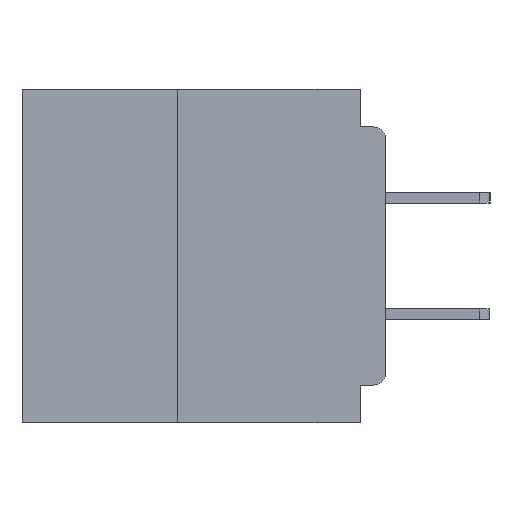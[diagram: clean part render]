
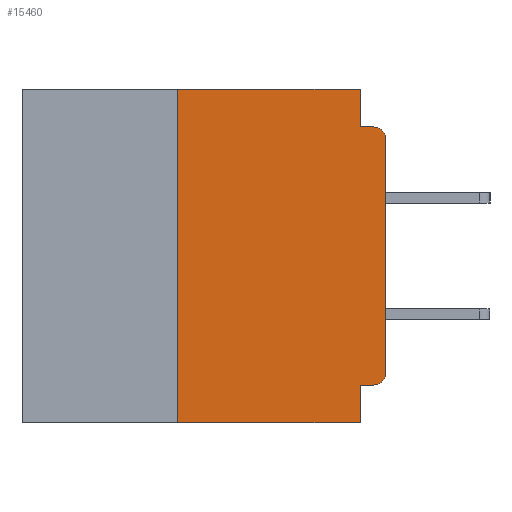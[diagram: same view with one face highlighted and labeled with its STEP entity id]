
A CAD part, left-side view. The second image highlights one B-rep face of the part: STEP entity #15460.
In plain terms, the highlighted planar face has unit normal (-1, 0, 0).
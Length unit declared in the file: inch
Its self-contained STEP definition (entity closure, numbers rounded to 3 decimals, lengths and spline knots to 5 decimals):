
#639 = EDGE_CURVE ( 'NONE', #4602, #40217, #16367, .T. ) ;
#1851 = ORIENTED_EDGE ( 'NONE', *, *, #38420, .F. ) ;
#2623 = LINE ( 'NONE', #29230, #11467 ) ;
#2652 = CARTESIAN_POINT ( 'NONE',  ( 0., 0.031, 0. ) ) ;
#2675 = CARTESIAN_POINT ( 'NONE',  ( 0., 0.015, -0.34 ) ) ;
#3031 = EDGE_CURVE ( 'NONE', #53284, #5341, #20967, .T. ) ;
#3651 = DIRECTION ( 'NONE',  ( 0., -1., 0. ) ) ;
#3928 = PLANE ( 'NONE',  #62300 ) ;
#4035 = DIRECTION ( 'NONE',  ( 0., 0., -1. ) ) ;
#4602 = VERTEX_POINT ( 'NONE', #41053 ) ;
#5341 = VERTEX_POINT ( 'NONE', #62107 ) ;
#5987 = ORIENTED_EDGE ( 'NONE', *, *, #14786, .F. ) ;
#6635 = ORIENTED_EDGE ( 'NONE', *, *, #27034, .F. ) ;
#7859 = DIRECTION ( 'NONE',  ( 0., 0., -1. ) ) ;
#7872 = EDGE_CURVE ( 'NONE', #63508, #13340, #45457, .T. ) ;
#8539 = DIRECTION ( 'NONE',  ( 0., 1., 0. ) ) ;
#9105 = DIRECTION ( 'NONE',  ( 0., 0., -1. ) ) ;
#9615 = LINE ( 'NONE', #51206, #62433 ) ;
#10127 = CARTESIAN_POINT ( 'NONE',  ( 0., 0.031, -0.4 ) ) ;
#11467 = VECTOR ( 'NONE', #3651, 39.37008 ) ;
#11957 = VECTOR ( 'NONE', #20599, 39.37008 ) ;
#12741 = CARTESIAN_POINT ( 'NONE',  ( 0., 0.25, -0.4 ) ) ;
#13340 = VERTEX_POINT ( 'NONE', #47732 ) ;
#14077 = CARTESIAN_POINT ( 'NONE',  ( 0., 0.437, 0. ) ) ;
#14786 = EDGE_CURVE ( 'NONE', #63508, #59188, #64488, .T. ) ;
#15460 = ADVANCED_FACE ( 'NONE', ( #37426 ), #3928, .F. ) ;
#15581 = VECTOR ( 'NONE', #4035, 39.37008 ) ;
#16317 = LINE ( 'NONE', #64250, #55476 ) ;
#16367 = LINE ( 'NONE', #40105, #26764 ) ;
#17853 = ORIENTED_EDGE ( 'NONE', *, *, #26024, .T. ) ;
#18044 = VECTOR ( 'NONE', #45025, 39.37008 ) ;
#18517 = DIRECTION ( 'NONE',  ( 0., 0., -1. ) ) ;
#18874 = VERTEX_POINT ( 'NONE', #64544 ) ;
#18918 = AXIS2_PLACEMENT_3D ( 'NONE', #51100, #20511, #56238 ) ;
#19669 = EDGE_CURVE ( 'NONE', #59188, #24117, #22003, .T. ) ;
#20363 = ORIENTED_EDGE ( 'NONE', *, *, #22897, .T. ) ;
#20511 = DIRECTION ( 'NONE',  ( -1., 0., 0. ) ) ;
#20599 = DIRECTION ( 'NONE',  ( 0., -1., 0. ) ) ;
#20967 = CIRCLE ( 'NONE', #18918, 0.015 ) ;
#22003 = LINE ( 'NONE', #45058, #15581 ) ;
#22897 = EDGE_CURVE ( 'NONE', #30338, #24117, #63167, .T. ) ;
#22945 = CARTESIAN_POINT ( 'NONE',  ( 0., 0.015, -0.355 ) ) ;
#24117 = VERTEX_POINT ( 'NONE', #10127 ) ;
#25753 = DIRECTION ( 'NONE',  ( 0., 0., 1. ) ) ;
#26024 = EDGE_CURVE ( 'NONE', #13340, #53284, #58818, .T. ) ;
#26764 = VECTOR ( 'NONE', #40774, 39.37008 ) ;
#26951 = EDGE_CURVE ( 'NONE', #40217, #18874, #16317, .T. ) ;
#27034 = EDGE_CURVE ( 'NONE', #18874, #5341, #2623, .T. ) ;
#29230 = CARTESIAN_POINT ( 'NONE',  ( 0., 0., -0.045 ) ) ;
#30338 = VERTEX_POINT ( 'NONE', #12741 ) ;
#30377 = CARTESIAN_POINT ( 'NONE',  ( 0., 0., -0.06 ) ) ;
#34748 = ORIENTED_EDGE ( 'NONE', *, *, #639, .F. ) ;
#34998 = AXIS2_PLACEMENT_3D ( 'NONE', #2675, #38575, #7859 ) ;
#37426 = FACE_OUTER_BOUND ( 'NONE', #39822, .T. ) ;
#38420 = EDGE_CURVE ( 'NONE', #30338, #4602, #9615, .T. ) ;
#38575 = DIRECTION ( 'NONE',  ( -1., 0., 0. ) ) ;
#39017 = VECTOR ( 'NONE', #8539, 39.37008 ) ;
#39250 = CARTESIAN_POINT ( 'NONE',  ( 0., 0., -0.355 ) ) ;
#39822 = EDGE_LOOP ( 'NONE', ( #17853, #42738, #6635, #40343, #34748, #1851, #20363, #43602, #5987, #46840 ) ) ;
#39840 = DIRECTION ( 'NONE',  ( 1., 0., 0. ) ) ;
#40105 = CARTESIAN_POINT ( 'NONE',  ( 0., 0.437, 0. ) ) ;
#40217 = VERTEX_POINT ( 'NONE', #2652 ) ;
#40343 = ORIENTED_EDGE ( 'NONE', *, *, #26951, .F. ) ;
#40774 = DIRECTION ( 'NONE',  ( 0., -1., 0. ) ) ;
#41053 = CARTESIAN_POINT ( 'NONE',  ( 0., 0.25, 0. ) ) ;
#42738 = ORIENTED_EDGE ( 'NONE', *, *, #3031, .T. ) ;
#43602 = ORIENTED_EDGE ( 'NONE', *, *, #19669, .F. ) ;
#45025 = DIRECTION ( 'NONE',  ( 0., 0., 1. ) ) ;
#45058 = CARTESIAN_POINT ( 'NONE',  ( 0., 0.031, -0.4 ) ) ;
#45457 = CIRCLE ( 'NONE', #34998, 0.015 ) ;
#46063 = CARTESIAN_POINT ( 'NONE',  ( 0., 0.437, -0.4 ) ) ;
#46840 = ORIENTED_EDGE ( 'NONE', *, *, #7872, .T. ) ;
#47732 = CARTESIAN_POINT ( 'NONE',  ( 0., 0., -0.34 ) ) ;
#51100 = CARTESIAN_POINT ( 'NONE',  ( 0., 0.015, -0.06 ) ) ;
#51206 = CARTESIAN_POINT ( 'NONE',  ( 0., 0.25, -0.4 ) ) ;
#53284 = VERTEX_POINT ( 'NONE', #30377 ) ;
#55476 = VECTOR ( 'NONE', #18517, 39.37008 ) ;
#56238 = DIRECTION ( 'NONE',  ( 0., 0., -1. ) ) ;
#58818 = LINE ( 'NONE', #60615, #18044 ) ;
#59188 = VERTEX_POINT ( 'NONE', #65979 ) ;
#60615 = CARTESIAN_POINT ( 'NONE',  ( 0., 0., 0. ) ) ;
#62107 = CARTESIAN_POINT ( 'NONE',  ( 0., 0.015, -0.045 ) ) ;
#62300 = AXIS2_PLACEMENT_3D ( 'NONE', #14077, #39840, #9105 ) ;
#62433 = VECTOR ( 'NONE', #25753, 39.37008 ) ;
#63167 = LINE ( 'NONE', #46063, #11957 ) ;
#63508 = VERTEX_POINT ( 'NONE', #22945 ) ;
#64250 = CARTESIAN_POINT ( 'NONE',  ( 0., 0.031, 0. ) ) ;
#64488 = LINE ( 'NONE', #39250, #39017 ) ;
#64544 = CARTESIAN_POINT ( 'NONE',  ( 0., 0.031, -0.045 ) ) ;
#65979 = CARTESIAN_POINT ( 'NONE',  ( 0., 0.031, -0.355 ) ) ;
